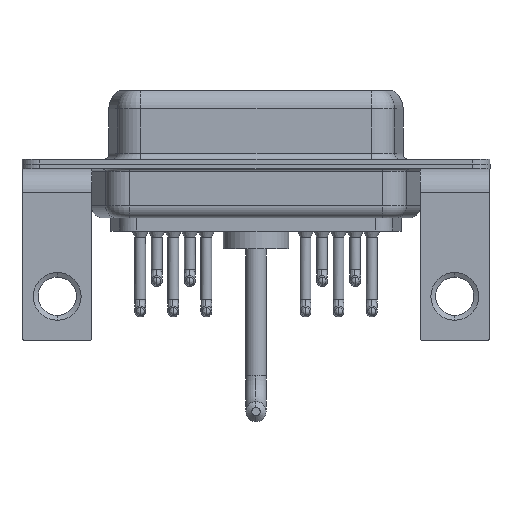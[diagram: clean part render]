
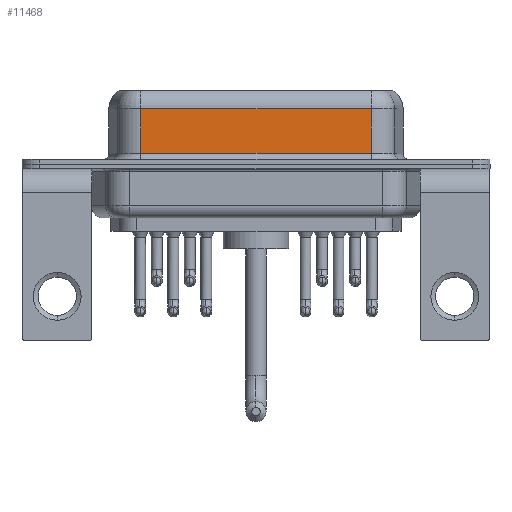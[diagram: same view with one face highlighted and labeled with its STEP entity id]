
A CAD part, front view. The second image highlights one B-rep face of the part: STEP entity #11468.
In plain terms, the highlighted planar face has unit normal (0, -1, 0).
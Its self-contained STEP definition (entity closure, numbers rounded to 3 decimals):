
#93 = FACE_OUTER_BOUND ( 'NONE', #18538, .T. ) ;
#295 = VECTOR ( 'NONE', #8062, 1000. ) ;
#575 = EDGE_CURVE ( 'NONE', #13036, #16914, #1157, .T. ) ;
#760 = VECTOR ( 'NONE', #13167, 1000. ) ;
#1157 = LINE ( 'NONE', #11771, #12809 ) ;
#1174 = CARTESIAN_POINT ( 'NONE',  ( 26.287, -3.95, 0.9 ) ) ;
#1935 = CARTESIAN_POINT ( 'NONE',  ( 7.013, -3.95, 0.9 ) ) ;
#2420 = CARTESIAN_POINT ( 'NONE',  ( 7.013, -3.95, 6.4 ) ) ;
#3456 = VECTOR ( 'NONE', #8403, 1000. ) ;
#4592 = DIRECTION ( 'NONE',  ( 0., 0., 1. ) ) ;
#4685 = CARTESIAN_POINT ( 'NONE',  ( 26.287, -3.95, 6.4 ) ) ;
#4687 = CARTESIAN_POINT ( 'NONE',  ( 26.287, -3.95, 0.9 ) ) ;
#5551 = EDGE_CURVE ( 'NONE', #13036, #10105, #17120, .T. ) ;
#5861 = ORIENTED_EDGE ( 'NONE', *, *, #6998, .T. ) ;
#6088 = PLANE ( 'NONE',  #12666 ) ;
#6551 = ORIENTED_EDGE ( 'NONE', *, *, #5551, .T. ) ;
#6998 = EDGE_CURVE ( 'NONE', #10105, #8228, #9887, .T. ) ;
#8062 = DIRECTION ( 'NONE',  ( -1., 0., 0. ) ) ;
#8228 = VERTEX_POINT ( 'NONE', #1935 ) ;
#8281 = CARTESIAN_POINT ( 'NONE',  ( 26.287, -3.95, 4.65 ) ) ;
#8403 = DIRECTION ( 'NONE',  ( 0., 0., -1. ) ) ;
#8628 = LINE ( 'NONE', #1174, #760 ) ;
#9887 = LINE ( 'NONE', #2420, #3456 ) ;
#10105 = VERTEX_POINT ( 'NONE', #17058 ) ;
#10726 = CARTESIAN_POINT ( 'NONE',  ( 26.287, -3.95, 4.65 ) ) ;
#11468 = ADVANCED_FACE ( 'NONE', ( #93 ), #6088, .F. ) ;
#11478 = DIRECTION ( 'NONE',  ( 0., 0., -1. ) ) ;
#11771 = CARTESIAN_POINT ( 'NONE',  ( 26.287, -3.95, 6.4 ) ) ;
#11817 = EDGE_CURVE ( 'NONE', #8228, #16914, #8628, .T. ) ;
#12666 = AXIS2_PLACEMENT_3D ( 'NONE', #4685, #18074, #4592 ) ;
#12809 = VECTOR ( 'NONE', #11478, 1000. ) ;
#13036 = VERTEX_POINT ( 'NONE', #8281 ) ;
#13167 = DIRECTION ( 'NONE',  ( 1., 0., 0. ) ) ;
#14545 = ORIENTED_EDGE ( 'NONE', *, *, #575, .F. ) ;
#16914 = VERTEX_POINT ( 'NONE', #4687 ) ;
#17058 = CARTESIAN_POINT ( 'NONE',  ( 7.013, -3.95, 4.65 ) ) ;
#17120 = LINE ( 'NONE', #10726, #295 ) ;
#17234 = ORIENTED_EDGE ( 'NONE', *, *, #11817, .T. ) ;
#18074 = DIRECTION ( 'NONE',  ( 0., 1., 0. ) ) ;
#18538 = EDGE_LOOP ( 'NONE', ( #14545, #6551, #5861, #17234 ) ) ;
